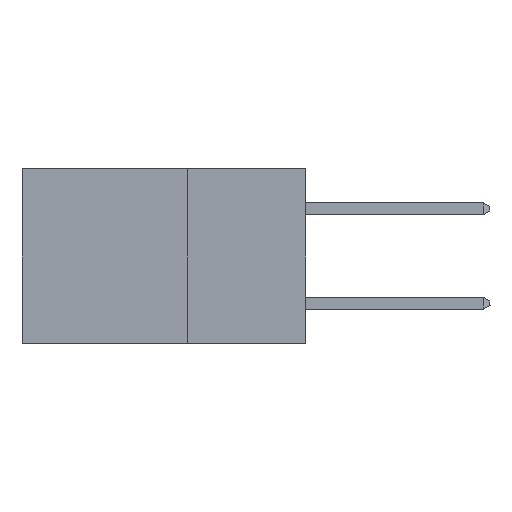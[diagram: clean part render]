
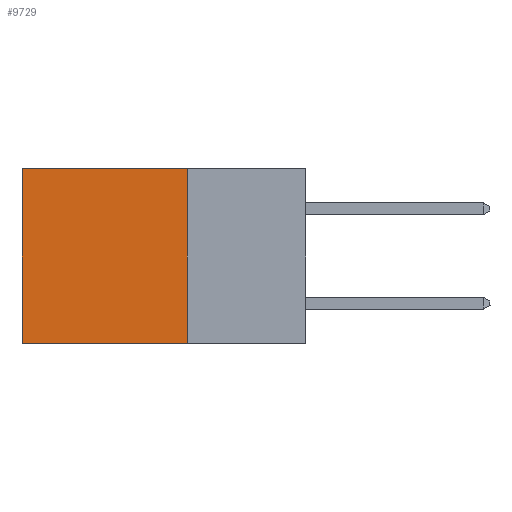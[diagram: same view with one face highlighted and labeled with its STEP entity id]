
A CAD part, left-side view. The second image highlights one B-rep face of the part: STEP entity #9729.
In plain terms, the highlighted planar face has unit normal (-1, 0, 0).
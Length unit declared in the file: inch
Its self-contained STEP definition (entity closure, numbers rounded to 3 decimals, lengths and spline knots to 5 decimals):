
#151 = PLANE ( 'NONE',  #6643 ) ;
#276 = CARTESIAN_POINT ( 'NONE',  ( 0.2615, 0.25, -0.37 ) ) ;
#612 = VERTEX_POINT ( 'NONE', #7399 ) ;
#967 = LINE ( 'NONE', #276, #8208 ) ;
#1664 = CARTESIAN_POINT ( 'NONE',  ( 0.2615, 0.6, -0.37 ) ) ;
#1805 = CARTESIAN_POINT ( 'NONE',  ( 0.2615, 0.6, -0.37 ) ) ;
#1885 = CARTESIAN_POINT ( 'NONE',  ( 0.2615, 0.25, 0. ) ) ;
#1998 = DIRECTION ( 'NONE',  ( 0., 1., 0. ) ) ;
#2092 = ORIENTED_EDGE ( 'NONE', *, *, #6023, .F. ) ;
#2246 = LINE ( 'NONE', #1885, #4986 ) ;
#2733 = EDGE_CURVE ( 'NONE', #3554, #9342, #10451, .T. ) ;
#2752 = CARTESIAN_POINT ( 'NONE',  ( 0.2615, 0.25, -0.37 ) ) ;
#2834 = DIRECTION ( 'NONE',  ( 0., 0., -1. ) ) ;
#3554 = VERTEX_POINT ( 'NONE', #8687 ) ;
#3630 = DIRECTION ( 'NONE',  ( 1., 0., 0. ) ) ;
#3887 = ORIENTED_EDGE ( 'NONE', *, *, #2733, .T. ) ;
#4986 = VECTOR ( 'NONE', #1998, 39.37008 ) ;
#5966 = VERTEX_POINT ( 'NONE', #10706 ) ;
#6023 = EDGE_CURVE ( 'NONE', #5966, #9342, #967, .T. ) ;
#6643 = AXIS2_PLACEMENT_3D ( 'NONE', #2752, #3630, #2834 ) ;
#6993 = DIRECTION ( 'NONE',  ( 0., 0., -1. ) ) ;
#7187 = FACE_OUTER_BOUND ( 'NONE', #9441, .T. ) ;
#7399 = CARTESIAN_POINT ( 'NONE',  ( 0.2615, 0.25, 0. ) ) ;
#7452 = LINE ( 'NONE', #10574, #8008 ) ;
#7977 = DIRECTION ( 'NONE',  ( 0., 1., 0. ) ) ;
#8008 = VECTOR ( 'NONE', #10509, 39.37008 ) ;
#8208 = VECTOR ( 'NONE', #7977, 39.37008 ) ;
#8687 = CARTESIAN_POINT ( 'NONE',  ( 0.2615, 0.6, 0. ) ) ;
#9342 = VERTEX_POINT ( 'NONE', #1664 ) ;
#9441 = EDGE_LOOP ( 'NONE', ( #3887, #2092, #10401, #11089 ) ) ;
#9492 = EDGE_CURVE ( 'NONE', #612, #5966, #7452, .T. ) ;
#9729 = ADVANCED_FACE ( 'NONE', ( #7187 ), #151, .F. ) ;
#9732 = EDGE_CURVE ( 'NONE', #612, #3554, #2246, .T. ) ;
#10025 = VECTOR ( 'NONE', #6993, 39.37008 ) ;
#10401 = ORIENTED_EDGE ( 'NONE', *, *, #9492, .F. ) ;
#10451 = LINE ( 'NONE', #1805, #10025 ) ;
#10509 = DIRECTION ( 'NONE',  ( 0., 0., -1. ) ) ;
#10574 = CARTESIAN_POINT ( 'NONE',  ( 0.2615, 0.25, -0.37 ) ) ;
#10706 = CARTESIAN_POINT ( 'NONE',  ( 0.2615, 0.25, -0.37 ) ) ;
#11089 = ORIENTED_EDGE ( 'NONE', *, *, #9732, .T. ) ;
